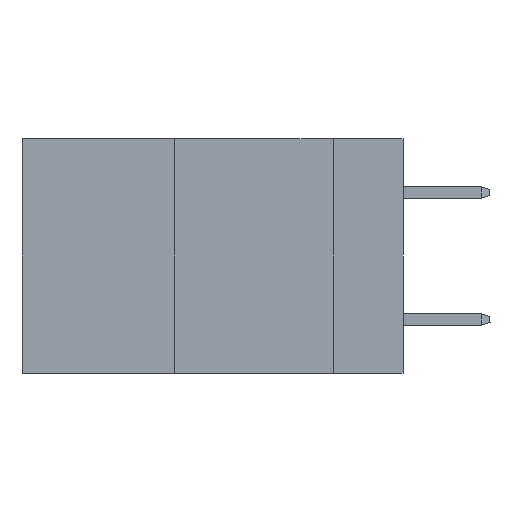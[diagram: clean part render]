
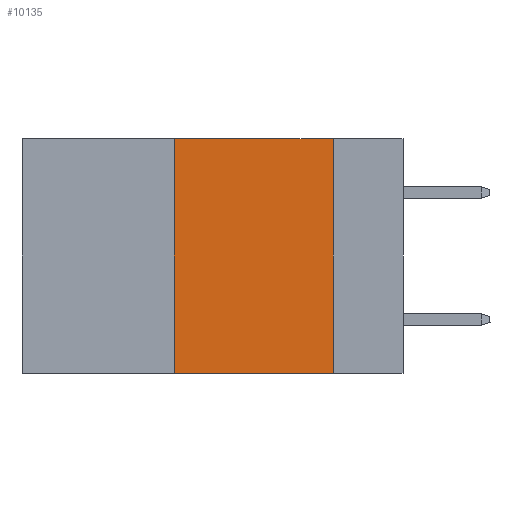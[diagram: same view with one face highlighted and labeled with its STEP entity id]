
A CAD part, left-side view. The second image highlights one B-rep face of the part: STEP entity #10135.
In plain terms, the highlighted planar face has unit normal (-1, 0, 0).
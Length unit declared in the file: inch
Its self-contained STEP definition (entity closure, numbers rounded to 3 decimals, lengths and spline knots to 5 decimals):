
#545 = FACE_OUTER_BOUND ( 'NONE', #2132, .T. ) ;
#1398 = ORIENTED_EDGE ( 'NONE', *, *, #12890, .F. ) ;
#1652 = CARTESIAN_POINT ( 'NONE',  ( 0., 0.36, 0. ) ) ;
#1871 = CARTESIAN_POINT ( 'NONE',  ( 0., 0.36, -0.37 ) ) ;
#2081 = LINE ( 'NONE', #13136, #6260 ) ;
#2132 = EDGE_LOOP ( 'NONE', ( #1398, #9330, #14344, #2316 ) ) ;
#2316 = ORIENTED_EDGE ( 'NONE', *, *, #5888, .T. ) ;
#2445 = VERTEX_POINT ( 'NONE', #4397 ) ;
#2647 = VECTOR ( 'NONE', #10584, 39.37008 ) ;
#2807 = LINE ( 'NONE', #5251, #14612 ) ;
#3021 = CARTESIAN_POINT ( 'NONE',  ( 0., 0.6, 0. ) ) ;
#4397 = CARTESIAN_POINT ( 'NONE',  ( 0., 0.11, -0.37 ) ) ;
#5115 = CARTESIAN_POINT ( 'NONE',  ( 0., 0.6, 0. ) ) ;
#5251 = CARTESIAN_POINT ( 'NONE',  ( 0., 0.6, -0.37 ) ) ;
#5583 = LINE ( 'NONE', #1652, #2647 ) ;
#5777 = DIRECTION ( 'NONE',  ( 1., 0., 0. ) ) ;
#5888 = EDGE_CURVE ( 'NONE', #12579, #2445, #2807, .T. ) ;
#6260 = VECTOR ( 'NONE', #7075, 39.37008 ) ;
#6325 = AXIS2_PLACEMENT_3D ( 'NONE', #3021, #5777, #15675 ) ;
#6594 = EDGE_CURVE ( 'NONE', #12803, #13345, #7489, .T. ) ;
#7075 = DIRECTION ( 'NONE',  ( 0., 0., -1. ) ) ;
#7185 = EDGE_CURVE ( 'NONE', #12579, #12803, #5583, .T. ) ;
#7489 = LINE ( 'NONE', #5115, #11535 ) ;
#7789 = DIRECTION ( 'NONE',  ( 0., -1., 0. ) ) ;
#9239 = PLANE ( 'NONE',  #6325 ) ;
#9330 = ORIENTED_EDGE ( 'NONE', *, *, #6594, .F. ) ;
#10111 = DIRECTION ( 'NONE',  ( 0., -1., 0. ) ) ;
#10135 = ADVANCED_FACE ( 'NONE', ( #545 ), #9239, .F. ) ;
#10532 = CARTESIAN_POINT ( 'NONE',  ( 0., 0.36, 0. ) ) ;
#10584 = DIRECTION ( 'NONE',  ( 0., 0., 1. ) ) ;
#11535 = VECTOR ( 'NONE', #10111, 39.37008 ) ;
#12579 = VERTEX_POINT ( 'NONE', #1871 ) ;
#12803 = VERTEX_POINT ( 'NONE', #10532 ) ;
#12890 = EDGE_CURVE ( 'NONE', #13345, #2445, #2081, .T. ) ;
#13136 = CARTESIAN_POINT ( 'NONE',  ( 0., 0.11, 0. ) ) ;
#13189 = CARTESIAN_POINT ( 'NONE',  ( 0., 0.11, 0. ) ) ;
#13345 = VERTEX_POINT ( 'NONE', #13189 ) ;
#14344 = ORIENTED_EDGE ( 'NONE', *, *, #7185, .F. ) ;
#14612 = VECTOR ( 'NONE', #7789, 39.37008 ) ;
#15675 = DIRECTION ( 'NONE',  ( 0., 0., -1. ) ) ;
